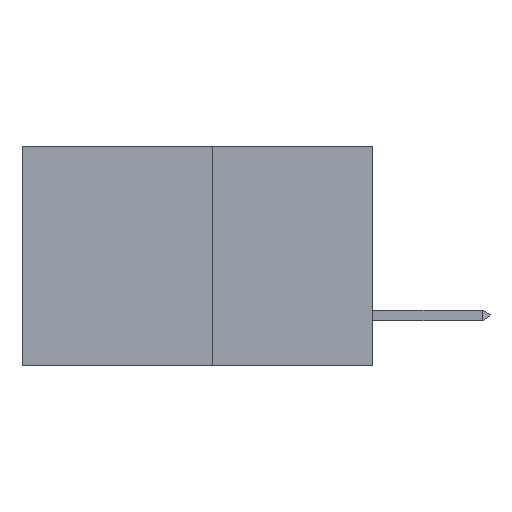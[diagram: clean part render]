
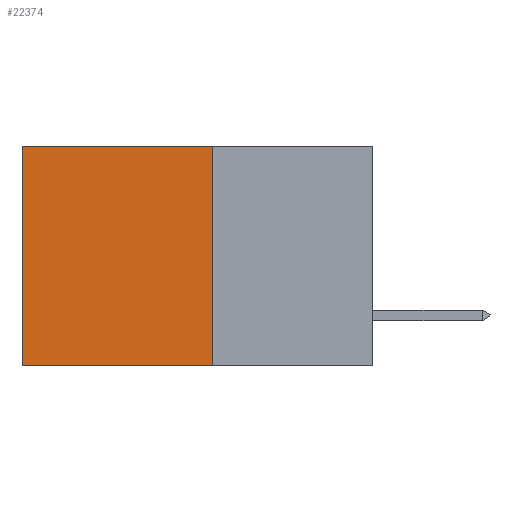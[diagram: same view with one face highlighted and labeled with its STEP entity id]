
A CAD part, left-side view. The second image highlights one B-rep face of the part: STEP entity #22374.
In plain terms, the highlighted planar face has unit normal (-1, 0, 0).
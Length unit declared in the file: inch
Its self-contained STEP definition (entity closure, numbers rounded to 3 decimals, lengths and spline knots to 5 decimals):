
#48 = EDGE_LOOP ( 'NONE', ( #10806, #14828, #10389, #7527 ) ) ;
#177 = AXIS2_PLACEMENT_3D ( 'NONE', #8390, #22119, #10387 ) ;
#1532 = VECTOR ( 'NONE', #11678, 39.37008 ) ;
#1898 = VERTEX_POINT ( 'NONE', #8823 ) ;
#2371 = LINE ( 'NONE', #6191, #12820 ) ;
#2742 = VERTEX_POINT ( 'NONE', #12627 ) ;
#2835 = LINE ( 'NONE', #3207, #17941 ) ;
#2947 = EDGE_CURVE ( 'NONE', #2742, #1898, #2371, .T. ) ;
#3074 = CARTESIAN_POINT ( 'NONE',  ( 0.277, 0.27, 0. ) ) ;
#3207 = CARTESIAN_POINT ( 'NONE',  ( 0.277, 0.27, -0.37 ) ) ;
#4550 = DIRECTION ( 'NONE',  ( 0., 0., -1. ) ) ;
#5349 = EDGE_CURVE ( 'NONE', #22561, #2742, #2835, .T. ) ;
#5388 = CARTESIAN_POINT ( 'NONE',  ( 0.277, 0.27, 0. ) ) ;
#6064 = DIRECTION ( 'NONE',  ( 0., 0., -1. ) ) ;
#6093 = DIRECTION ( 'NONE',  ( 0., 1., 0. ) ) ;
#6191 = CARTESIAN_POINT ( 'NONE',  ( 0.277, 0.27, -0.37 ) ) ;
#6278 = VECTOR ( 'NONE', #6064, 39.37008 ) ;
#6389 = CARTESIAN_POINT ( 'NONE',  ( 0.277, 0.59, -0.37 ) ) ;
#6709 = LINE ( 'NONE', #5388, #1532 ) ;
#7527 = ORIENTED_EDGE ( 'NONE', *, *, #8101, .T. ) ;
#7856 = VERTEX_POINT ( 'NONE', #8339 ) ;
#8101 = EDGE_CURVE ( 'NONE', #22561, #7856, #6709, .T. ) ;
#8339 = CARTESIAN_POINT ( 'NONE',  ( 0.277, 0.59, 0. ) ) ;
#8390 = CARTESIAN_POINT ( 'NONE',  ( 0.277, 0.27, -0.37 ) ) ;
#8823 = CARTESIAN_POINT ( 'NONE',  ( 0.277, 0.59, -0.37 ) ) ;
#10387 = DIRECTION ( 'NONE',  ( 0., 0., -1. ) ) ;
#10389 = ORIENTED_EDGE ( 'NONE', *, *, #5349, .F. ) ;
#10545 = EDGE_CURVE ( 'NONE', #7856, #1898, #16816, .T. ) ;
#10806 = ORIENTED_EDGE ( 'NONE', *, *, #10545, .T. ) ;
#11678 = DIRECTION ( 'NONE',  ( 0., 1., 0. ) ) ;
#12627 = CARTESIAN_POINT ( 'NONE',  ( 0.277, 0.27, -0.37 ) ) ;
#12820 = VECTOR ( 'NONE', #6093, 39.37008 ) ;
#14828 = ORIENTED_EDGE ( 'NONE', *, *, #2947, .F. ) ;
#16816 = LINE ( 'NONE', #6389, #6278 ) ;
#17941 = VECTOR ( 'NONE', #4550, 39.37008 ) ;
#18254 = PLANE ( 'NONE',  #177 ) ;
#22119 = DIRECTION ( 'NONE',  ( 1., 0., 0. ) ) ;
#22374 = ADVANCED_FACE ( 'NONE', ( #23963 ), #18254, .F. ) ;
#22561 = VERTEX_POINT ( 'NONE', #3074 ) ;
#23963 = FACE_OUTER_BOUND ( 'NONE', #48, .T. ) ;
